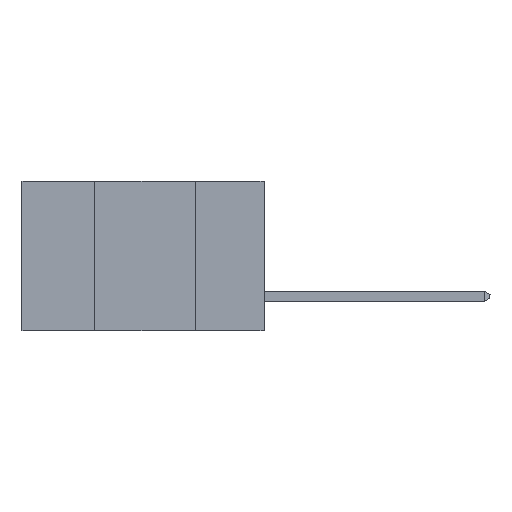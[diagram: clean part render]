
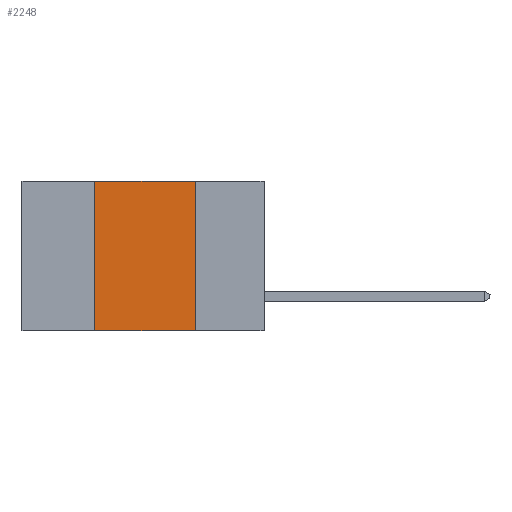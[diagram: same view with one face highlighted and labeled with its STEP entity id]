
A CAD part, left-side view. The second image highlights one B-rep face of the part: STEP entity #2248.
In plain terms, the highlighted planar face has unit normal (-1, 0, 0).
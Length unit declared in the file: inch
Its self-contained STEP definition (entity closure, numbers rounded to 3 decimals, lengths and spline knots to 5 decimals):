
#677 = CARTESIAN_POINT ( 'NONE',  ( 0., 0.17, 0. ) ) ;
#1121 = VERTEX_POINT ( 'NONE', #12664 ) ;
#1159 = VERTEX_POINT ( 'NONE', #14830 ) ;
#1570 = CARTESIAN_POINT ( 'NONE',  ( 0., 0.17, -0.37 ) ) ;
#2051 = VECTOR ( 'NONE', #12949, 39.37008 ) ;
#2172 = CARTESIAN_POINT ( 'NONE',  ( 0., 0.6, 0. ) ) ;
#2248 = ADVANCED_FACE ( 'NONE', ( #13151 ), #15304, .F. ) ;
#2316 = CARTESIAN_POINT ( 'NONE',  ( 0., 0.6, -0.37 ) ) ;
#2366 = EDGE_LOOP ( 'NONE', ( #3484, #7424, #14944, #14427 ) ) ;
#2455 = LINE ( 'NONE', #1570, #5747 ) ;
#2619 = DIRECTION ( 'NONE',  ( 0., 0., -1. ) ) ;
#3210 = DIRECTION ( 'NONE',  ( 1., 0., 0. ) ) ;
#3484 = ORIENTED_EDGE ( 'NONE', *, *, #7809, .F. ) ;
#5456 = VERTEX_POINT ( 'NONE', #11182 ) ;
#5747 = VECTOR ( 'NONE', #2619, 39.37008 ) ;
#6082 = EDGE_CURVE ( 'NONE', #1121, #5456, #7670, .T. ) ;
#6275 = VERTEX_POINT ( 'NONE', #677 ) ;
#6813 = DIRECTION ( 'NONE',  ( 0., 0., -1. ) ) ;
#7114 = LINE ( 'NONE', #2316, #10743 ) ;
#7194 = DIRECTION ( 'NONE',  ( 0., -1., 0. ) ) ;
#7424 = ORIENTED_EDGE ( 'NONE', *, *, #15349, .F. ) ;
#7670 = LINE ( 'NONE', #8799, #14517 ) ;
#7809 = EDGE_CURVE ( 'NONE', #6275, #1159, #2455, .T. ) ;
#8799 = CARTESIAN_POINT ( 'NONE',  ( 0., 0.42, -0.37 ) ) ;
#9903 = DIRECTION ( 'NONE',  ( 0., 0., 1. ) ) ;
#10438 = EDGE_CURVE ( 'NONE', #1121, #1159, #7114, .T. ) ;
#10743 = VECTOR ( 'NONE', #7194, 39.37008 ) ;
#11182 = CARTESIAN_POINT ( 'NONE',  ( 0., 0.42, 0. ) ) ;
#11271 = AXIS2_PLACEMENT_3D ( 'NONE', #2172, #3210, #6813 ) ;
#12664 = CARTESIAN_POINT ( 'NONE',  ( 0., 0.42, -0.37 ) ) ;
#12949 = DIRECTION ( 'NONE',  ( 0., -1., 0. ) ) ;
#13121 = CARTESIAN_POINT ( 'NONE',  ( 0., 0.6, 0. ) ) ;
#13151 = FACE_OUTER_BOUND ( 'NONE', #2366, .T. ) ;
#13259 = LINE ( 'NONE', #13121, #2051 ) ;
#14427 = ORIENTED_EDGE ( 'NONE', *, *, #10438, .T. ) ;
#14517 = VECTOR ( 'NONE', #9903, 39.37008 ) ;
#14830 = CARTESIAN_POINT ( 'NONE',  ( 0., 0.17, -0.37 ) ) ;
#14944 = ORIENTED_EDGE ( 'NONE', *, *, #6082, .F. ) ;
#15304 = PLANE ( 'NONE',  #11271 ) ;
#15349 = EDGE_CURVE ( 'NONE', #5456, #6275, #13259, .T. ) ;
